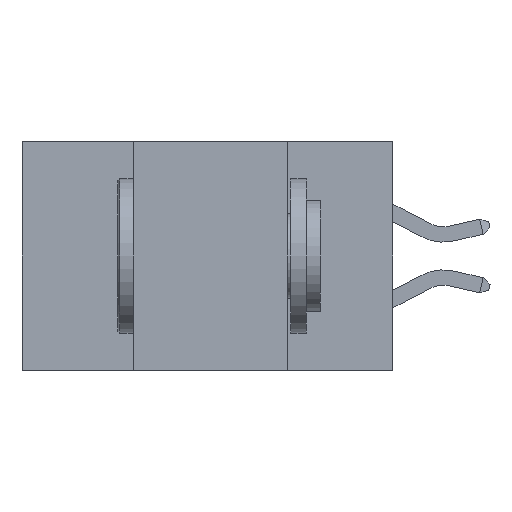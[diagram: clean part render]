
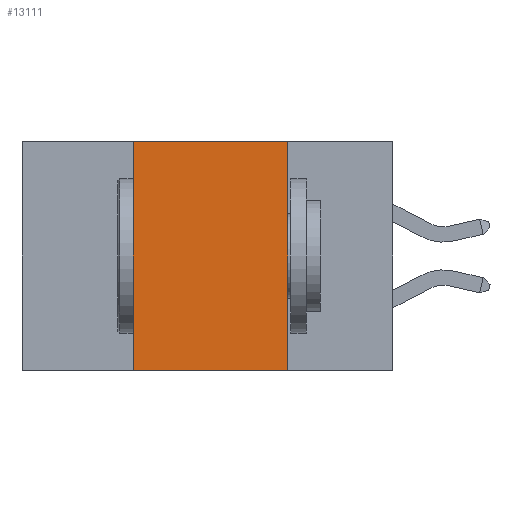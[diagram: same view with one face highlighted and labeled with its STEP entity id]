
A CAD part, left-side view. The second image highlights one B-rep face of the part: STEP entity #13111.
In plain terms, the highlighted planar face has unit normal (-1, 0, 0).
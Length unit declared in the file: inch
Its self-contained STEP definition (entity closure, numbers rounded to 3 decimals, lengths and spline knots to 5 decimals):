
#294 = VERTEX_POINT ( 'NONE', #19810 ) ;
#425 = CARTESIAN_POINT ( 'NONE',  ( 0., 0.6, -0.37 ) ) ;
#2678 = DIRECTION ( 'NONE',  ( 0., -1., 0. ) ) ;
#3053 = LINE ( 'NONE', #17757, #12841 ) ;
#6115 = ORIENTED_EDGE ( 'NONE', *, *, #14223, .T. ) ;
#6586 = DIRECTION ( 'NONE',  ( 1., 0., 0. ) ) ;
#7015 = CARTESIAN_POINT ( 'NONE',  ( 0., 0.42, 0. ) ) ;
#7665 = EDGE_CURVE ( 'NONE', #294, #15446, #3053, .T. ) ;
#8028 = DIRECTION ( 'NONE',  ( 0., 0., 1. ) ) ;
#8479 = VECTOR ( 'NONE', #15194, 39.37008 ) ;
#9042 = LINE ( 'NONE', #425, #8479 ) ;
#10432 = VERTEX_POINT ( 'NONE', #14386 ) ;
#11223 = VECTOR ( 'NONE', #2678, 39.37008 ) ;
#11455 = ORIENTED_EDGE ( 'NONE', *, *, #7665, .F. ) ;
#11700 = AXIS2_PLACEMENT_3D ( 'NONE', #17405, #6586, #19170 ) ;
#12314 = VECTOR ( 'NONE', #8028, 39.37008 ) ;
#12432 = EDGE_CURVE ( 'NONE', #12632, #294, #20110, .T. ) ;
#12632 = VERTEX_POINT ( 'NONE', #7015 ) ;
#12841 = VECTOR ( 'NONE', #19435, 39.37008 ) ;
#13111 = ADVANCED_FACE ( 'NONE', ( #19962 ), #19090, .F. ) ;
#13261 = ORIENTED_EDGE ( 'NONE', *, *, #12432, .F. ) ;
#13755 = EDGE_LOOP ( 'NONE', ( #11455, #13261, #18879, #6115 ) ) ;
#14223 = EDGE_CURVE ( 'NONE', #10432, #15446, #9042, .T. ) ;
#14386 = CARTESIAN_POINT ( 'NONE',  ( 0., 0.42, -0.37 ) ) ;
#15194 = DIRECTION ( 'NONE',  ( 0., -1., 0. ) ) ;
#15446 = VERTEX_POINT ( 'NONE', #18445 ) ;
#17405 = CARTESIAN_POINT ( 'NONE',  ( 0., 0.6, 0. ) ) ;
#17757 = CARTESIAN_POINT ( 'NONE',  ( 0., 0.17, 0. ) ) ;
#18445 = CARTESIAN_POINT ( 'NONE',  ( 0., 0.17, -0.37 ) ) ;
#18879 = ORIENTED_EDGE ( 'NONE', *, *, #22435, .F. ) ;
#19038 = CARTESIAN_POINT ( 'NONE',  ( 0., 0.6, 0. ) ) ;
#19090 = PLANE ( 'NONE',  #11700 ) ;
#19170 = DIRECTION ( 'NONE',  ( 0., 0., -1. ) ) ;
#19435 = DIRECTION ( 'NONE',  ( 0., 0., -1. ) ) ;
#19810 = CARTESIAN_POINT ( 'NONE',  ( 0., 0.17, 0. ) ) ;
#19962 = FACE_OUTER_BOUND ( 'NONE', #13755, .T. ) ;
#20062 = LINE ( 'NONE', #20548, #12314 ) ;
#20110 = LINE ( 'NONE', #19038, #11223 ) ;
#20548 = CARTESIAN_POINT ( 'NONE',  ( 0., 0.42, 0. ) ) ;
#22435 = EDGE_CURVE ( 'NONE', #10432, #12632, #20062, .T. ) ;
